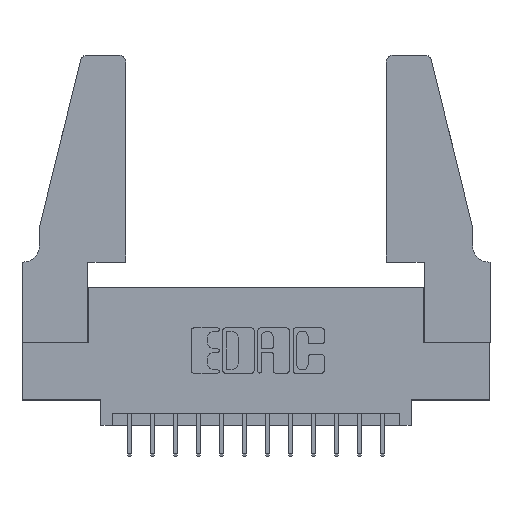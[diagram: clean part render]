
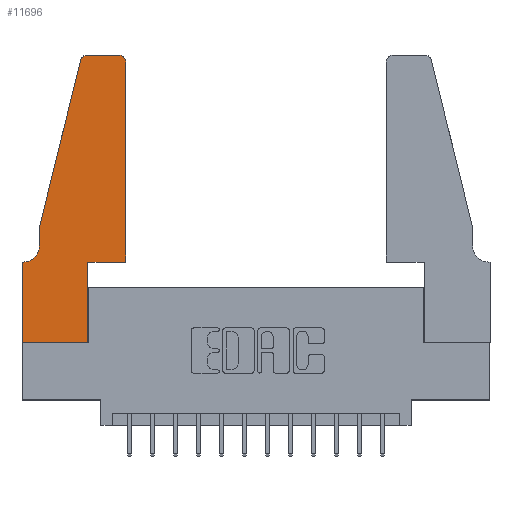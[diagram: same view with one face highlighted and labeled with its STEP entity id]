
A CAD part, top view. The second image highlights one B-rep face of the part: STEP entity #11696.
In plain terms, the highlighted planar face has unit normal (0, 0, 1).
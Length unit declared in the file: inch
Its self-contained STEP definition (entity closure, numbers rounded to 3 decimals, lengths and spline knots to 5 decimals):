
#156 = CARTESIAN_POINT ( 'NONE',  ( 0.4505, 0.35, 0.37 ) ) ;
#286 = AXIS2_PLACEMENT_3D ( 'NONE', #766, #8155, #9345 ) ;
#380 = CARTESIAN_POINT ( 'NONE',  ( 0.2605, 1.25, 0.37 ) ) ;
#488 = CARTESIAN_POINT ( 'NONE',  ( 0.0755, 0.42, 0.37 ) ) ;
#520 = EDGE_CURVE ( 'NONE', #11193, #3086, #7717, .T. ) ;
#542 = VERTEX_POINT ( 'NONE', #488 ) ;
#674 = CIRCLE ( 'NONE', #1178, 0.03 ) ;
#766 = CARTESIAN_POINT ( 'NONE',  ( 0., 0.35, 0.37 ) ) ;
#774 = VERTEX_POINT ( 'NONE', #1516 ) ;
#975 = DIRECTION ( 'NONE',  ( 1., 0., 0. ) ) ;
#991 = EDGE_CURVE ( 'NONE', #542, #11554, #12046, .T. ) ;
#1004 = VECTOR ( 'NONE', #8390, 39.37008 ) ;
#1178 = AXIS2_PLACEMENT_3D ( 'NONE', #6119, #14757, #8592 ) ;
#1255 = VECTOR ( 'NONE', #8205, 39.37008 ) ;
#1316 = CARTESIAN_POINT ( 'NONE',  ( 0.2865, 0.35, 0.37 ) ) ;
#1516 = CARTESIAN_POINT ( 'NONE',  ( 0.4205, 1.25, 0.37 ) ) ;
#1630 = DIRECTION ( 'NONE',  ( 0., 0., 1. ) ) ;
#1710 = DIRECTION ( 'NONE',  ( -1., 0., 0. ) ) ;
#2750 = ORIENTED_EDGE ( 'NONE', *, *, #9850, .T. ) ;
#2871 = CARTESIAN_POINT ( 'NONE',  ( 0.4505, 0.35, 0.37 ) ) ;
#3086 = VERTEX_POINT ( 'NONE', #6788 ) ;
#3386 = ORIENTED_EDGE ( 'NONE', *, *, #7640, .T. ) ;
#3446 = CARTESIAN_POINT ( 'NONE',  ( 0., 0., 0.37 ) ) ;
#3509 = CARTESIAN_POINT ( 'NONE',  ( 0.25487, 1.22718, 0.37 ) ) ;
#3723 = VERTEX_POINT ( 'NONE', #5528 ) ;
#3785 = LINE ( 'NONE', #10205, #12732 ) ;
#3940 = VERTEX_POINT ( 'NONE', #6018 ) ;
#4609 = ORIENTED_EDGE ( 'NONE', *, *, #9082, .T. ) ;
#4625 = CIRCLE ( 'NONE', #13084, 0.03 ) ;
#4671 = CARTESIAN_POINT ( 'NONE',  ( 0., 0.35, 0.37 ) ) ;
#4997 = EDGE_CURVE ( 'NONE', #13270, #5542, #674, .T. ) ;
#5063 = LINE ( 'NONE', #6109, #13189 ) ;
#5128 = DIRECTION ( 'NONE',  ( 1., 0., 0. ) ) ;
#5293 = DIRECTION ( 'NONE',  ( -1., 0., 0. ) ) ;
#5528 = CARTESIAN_POINT ( 'NONE',  ( 0.2865, 0., 0.37 ) ) ;
#5542 = VERTEX_POINT ( 'NONE', #3509 ) ;
#5663 = DIRECTION ( 'NONE',  ( 0., -1., 0. ) ) ;
#5749 = LINE ( 'NONE', #8138, #6925 ) ;
#5776 = VECTOR ( 'NONE', #10043, 39.37008 ) ;
#5823 = LINE ( 'NONE', #3446, #6913 ) ;
#5891 = CARTESIAN_POINT ( 'NONE',  ( 0.4505, 0.35, 0.37 ) ) ;
#6018 = CARTESIAN_POINT ( 'NONE',  ( 0., 0., 0.37 ) ) ;
#6109 = CARTESIAN_POINT ( 'NONE',  ( 0.0755, 0.5, 0.37 ) ) ;
#6119 = CARTESIAN_POINT ( 'NONE',  ( 0.284, 1.22, 0.37 ) ) ;
#6127 = EDGE_CURVE ( 'NONE', #11554, #7612, #3785, .T. ) ;
#6374 = EDGE_LOOP ( 'NONE', ( #14605, #7468, #7314, #10243, #15149, #7947, #2750, #3386, #9311, #4609, #12048, #14145 ) ) ;
#6488 = LINE ( 'NONE', #380, #7233 ) ;
#6788 = CARTESIAN_POINT ( 'NONE',  ( 0.4505, 1.22, 0.37 ) ) ;
#6837 = VERTEX_POINT ( 'NONE', #10380 ) ;
#6913 = VECTOR ( 'NONE', #975, 39.37008 ) ;
#6925 = VECTOR ( 'NONE', #5663, 39.37008 ) ;
#7233 = VECTOR ( 'NONE', #5293, 39.37008 ) ;
#7314 = ORIENTED_EDGE ( 'NONE', *, *, #14646, .T. ) ;
#7468 = ORIENTED_EDGE ( 'NONE', *, *, #4997, .T. ) ;
#7598 = CARTESIAN_POINT ( 'NONE',  ( 0.0055, 0.42, 0.37 ) ) ;
#7612 = VERTEX_POINT ( 'NONE', #4671 ) ;
#7640 = EDGE_CURVE ( 'NONE', #3940, #3723, #5823, .T. ) ;
#7717 = LINE ( 'NONE', #2871, #5776 ) ;
#7737 = CARTESIAN_POINT ( 'NONE',  ( 0.284, 1.25, 0.37 ) ) ;
#7947 = ORIENTED_EDGE ( 'NONE', *, *, #6127, .T. ) ;
#8138 = CARTESIAN_POINT ( 'NONE',  ( 0., 0., 0.37 ) ) ;
#8155 = DIRECTION ( 'NONE',  ( 0., 0., 1. ) ) ;
#8205 = DIRECTION ( 'NONE',  ( 1., 0., 0. ) ) ;
#8390 = DIRECTION ( 'NONE',  ( 0., 1., 0. ) ) ;
#8407 = CARTESIAN_POINT ( 'NONE',  ( 0.0055, 0.35, 0.37 ) ) ;
#8592 = DIRECTION ( 'NONE',  ( 1., 0., 0. ) ) ;
#8638 = CARTESIAN_POINT ( 'NONE',  ( 0.2865, 0.35, 0.37 ) ) ;
#9082 = EDGE_CURVE ( 'NONE', #11822, #11193, #10823, .T. ) ;
#9102 = DIRECTION ( 'NONE',  ( 0., 0., -1. ) ) ;
#9262 = PLANE ( 'NONE',  #286 ) ;
#9311 = ORIENTED_EDGE ( 'NONE', *, *, #9754, .T. ) ;
#9345 = DIRECTION ( 'NONE',  ( 1., 0., 0. ) ) ;
#9697 = LINE ( 'NONE', #11051, #14196 ) ;
#9754 = EDGE_CURVE ( 'NONE', #3723, #11822, #11996, .T. ) ;
#9850 = EDGE_CURVE ( 'NONE', #7612, #3940, #5749, .T. ) ;
#9851 = DIRECTION ( 'NONE',  ( -0.239, -0.971, 0. ) ) ;
#9934 = DIRECTION ( 'NONE',  ( 0., -1., 0. ) ) ;
#10043 = DIRECTION ( 'NONE',  ( 0., 1., 0. ) ) ;
#10205 = CARTESIAN_POINT ( 'NONE',  ( 0.0755, 0.35, 0.37 ) ) ;
#10243 = ORIENTED_EDGE ( 'NONE', *, *, #14598, .T. ) ;
#10380 = CARTESIAN_POINT ( 'NONE',  ( 0.0755, 0.5, 0.37 ) ) ;
#10823 = LINE ( 'NONE', #5891, #1255 ) ;
#11051 = CARTESIAN_POINT ( 'NONE',  ( 0.0755, 0.5, 0.37 ) ) ;
#11193 = VERTEX_POINT ( 'NONE', #156 ) ;
#11335 = CARTESIAN_POINT ( 'NONE',  ( 0.4205, 1.22, 0.37 ) ) ;
#11554 = VERTEX_POINT ( 'NONE', #8407 ) ;
#11595 = EDGE_CURVE ( 'NONE', #3086, #774, #4625, .T. ) ;
#11696 = ADVANCED_FACE ( 'NONE', ( #11831 ), #9262, .T. ) ;
#11822 = VERTEX_POINT ( 'NONE', #8638 ) ;
#11831 = FACE_OUTER_BOUND ( 'NONE', #6374, .T. ) ;
#11996 = LINE ( 'NONE', #1316, #1004 ) ;
#12046 = CIRCLE ( 'NONE', #14599, 0.07 ) ;
#12048 = ORIENTED_EDGE ( 'NONE', *, *, #520, .T. ) ;
#12480 = EDGE_CURVE ( 'NONE', #774, #13270, #6488, .T. ) ;
#12732 = VECTOR ( 'NONE', #12768, 39.37008 ) ;
#12768 = DIRECTION ( 'NONE',  ( -1., 0., 0. ) ) ;
#13084 = AXIS2_PLACEMENT_3D ( 'NONE', #11335, #1630, #5128 ) ;
#13189 = VECTOR ( 'NONE', #9934, 39.37008 ) ;
#13270 = VERTEX_POINT ( 'NONE', #7737 ) ;
#14145 = ORIENTED_EDGE ( 'NONE', *, *, #11595, .T. ) ;
#14196 = VECTOR ( 'NONE', #9851, 39.37008 ) ;
#14598 = EDGE_CURVE ( 'NONE', #6837, #542, #5063, .T. ) ;
#14599 = AXIS2_PLACEMENT_3D ( 'NONE', #7598, #9102, #1710 ) ;
#14605 = ORIENTED_EDGE ( 'NONE', *, *, #12480, .T. ) ;
#14646 = EDGE_CURVE ( 'NONE', #5542, #6837, #9697, .T. ) ;
#14757 = DIRECTION ( 'NONE',  ( 0., 0., 1. ) ) ;
#15149 = ORIENTED_EDGE ( 'NONE', *, *, #991, .T. ) ;
